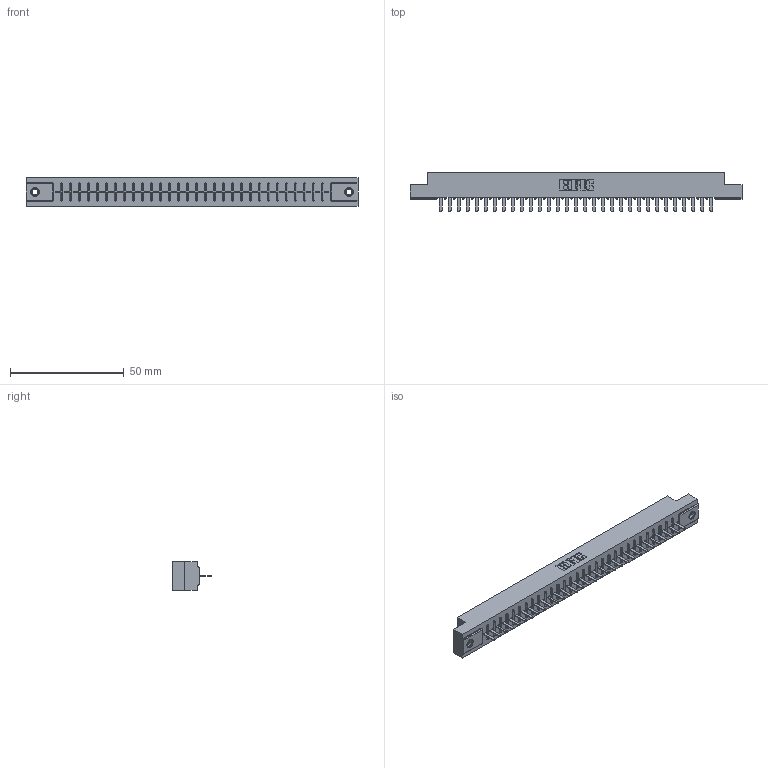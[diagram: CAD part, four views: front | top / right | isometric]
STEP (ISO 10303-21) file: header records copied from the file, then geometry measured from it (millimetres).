
FILE_DESCRIPTION (( 'STEP AP203' ), '1' );
FILE_NAME ('356-031-520-107.STEP', '2018-08-01T21:06:48', ( '' ), ( '' ), 'SwSTEP 2.0', 'SolidWorks 2016', '' );
FILE_SCHEMA (( 'CONFIG_CONTROL_DESIGN' ));
Length unit declared in the file: inch
Products named in the file (4): 306 Part_.156 Dia; 306-290-001_120; 345-250-001_345-250-005-103; 356-031-520-107
Assembly tree (34 placements, depth 2):
  356-031-520-107
    306 Part_.156 Dia
    306-290-001_120  x31
    345-250-001_345-250-005-103  x2
Bounding box: 145.85 x 17.12 x 12.7 mm (x, y, z)
Volume: 16017 mm3; surface area: 16372.9 mm2
Topology: 34 solids, 34 shells, 2346 faces, 6559 edges, 4198 vertices
Faces by surface type: plane 1557, cylinder 649, sphere 124, cone 12, torus 4
Entity records: 31475 total; most frequent: CARTESIAN_POINT 5263, ORIENTED_EDGE 5210, DIRECTION 5199, EDGE_CURVE 2605, LINE 2031, VECTOR 2031, VERTEX_POINT 1648, AXIS2_PLACEMENT_3D 1584
